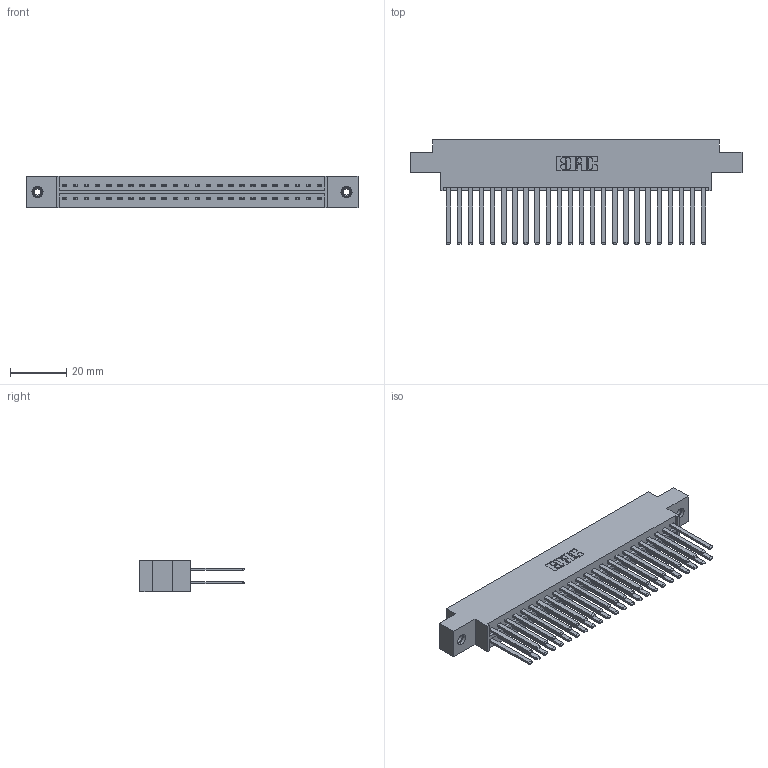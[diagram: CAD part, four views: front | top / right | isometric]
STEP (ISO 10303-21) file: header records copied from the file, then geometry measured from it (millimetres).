
FILE_DESCRIPTION (( 'STEP AP203' ), '1' );
FILE_NAME ('336-048-541-808.STEP', '2020-08-08T00:05:09', ( '' ), ( '' ), 'SwSTEP 2.0', 'SolidWorks 2020', '' );
FILE_SCHEMA (( 'CONFIG_CONTROL_DESIGN' ));
Length unit declared in the file: inch
Products named in the file (4): 336-290-001_336-290-541; 345-250-001_345-250-003-102; 336 Part_Offset - .156 Dia - TI; 336-048-541-808
Assembly tree (51 placements, depth 2):
  336-048-541-808
    336 Part_Offset - .156 Dia - TI
    336-290-001_336-290-541  x48
    345-250-001_345-250-003-102  x2
Bounding box: 118.49 x 37.34 x 11.1 mm (x, y, z)
Volume: 17710.2 mm3; surface area: 22395.8 mm2
Topology: 51 solids, 51 shells, 2194 faces, 6555 edges, 4330 vertices
Faces by surface type: plane 1354, cylinder 824, cone 12, torus 4
Entity records: 21973 total; most frequent: CARTESIAN_POINT 3780, ORIENTED_EDGE 3610, DIRECTION 3183, EDGE_CURVE 1805, LINE 1653, VECTOR 1653, VERTEX_POINT 1198, AXIS2_PLACEMENT_3D 765
